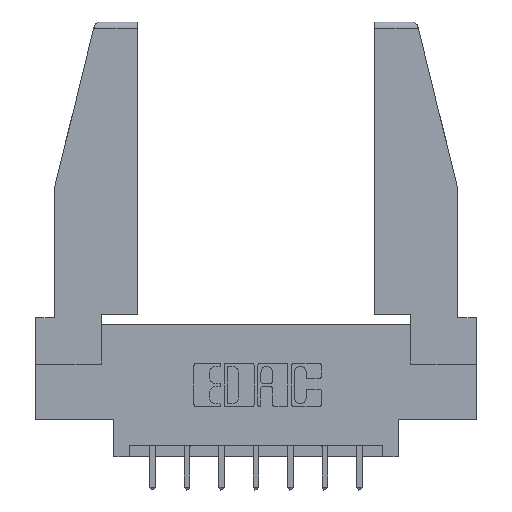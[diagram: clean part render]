
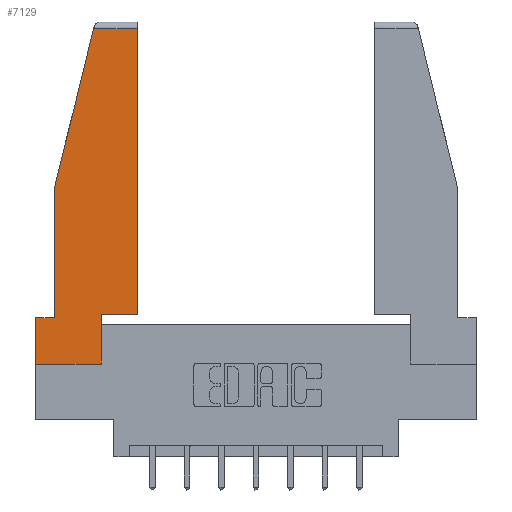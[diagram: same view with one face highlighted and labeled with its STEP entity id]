
A CAD part, top view. The second image highlights one B-rep face of the part: STEP entity #7129.
In plain terms, the highlighted planar face has unit normal (0, 0, 1).
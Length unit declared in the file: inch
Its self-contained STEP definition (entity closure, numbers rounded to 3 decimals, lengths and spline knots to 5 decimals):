
#118 = EDGE_CURVE ( 'NONE', #1076, #5311, #9170, .T. ) ;
#163 = VERTEX_POINT ( 'NONE', #5071 ) ;
#207 = VERTEX_POINT ( 'NONE', #1488 ) ;
#299 = VERTEX_POINT ( 'NONE', #12208 ) ;
#421 = CARTESIAN_POINT ( 'NONE',  ( 0.297, 0., 0. ) ) ;
#487 = VECTOR ( 'NONE', #8789, 39.37008 ) ;
#527 = AXIS2_PLACEMENT_3D ( 'NONE', #10409, #12367, #9402 ) ;
#644 = ORIENTED_EDGE ( 'NONE', *, *, #118, .T. ) ;
#921 = VERTEX_POINT ( 'NONE', #3981 ) ;
#1009 = ORIENTED_EDGE ( 'NONE', *, *, #2894, .T. ) ;
#1076 = VERTEX_POINT ( 'NONE', #8357 ) ;
#1488 = CARTESIAN_POINT ( 'NONE',  ( 0.297, 0., 0. ) ) ;
#1606 = VECTOR ( 'NONE', #11080, 39.37008 ) ;
#1769 = LINE ( 'NONE', #5513, #10834 ) ;
#1912 = VERTEX_POINT ( 'NONE', #5846 ) ;
#2113 = DIRECTION ( 'NONE',  ( 1., 0., 0. ) ) ;
#2365 = DIRECTION ( 'NONE',  ( 0., 1., 0. ) ) ;
#2510 = CARTESIAN_POINT ( 'NONE',  ( 0.461, 1.52, 0. ) ) ;
#2894 = EDGE_CURVE ( 'NONE', #207, #1076, #9684, .T. ) ;
#2986 = ORIENTED_EDGE ( 'NONE', *, *, #12083, .T. ) ;
#3292 = ORIENTED_EDGE ( 'NONE', *, *, #3628, .T. ) ;
#3396 = EDGE_CURVE ( 'NONE', #299, #207, #4759, .T. ) ;
#3402 = VECTOR ( 'NONE', #2113, 39.37008 ) ;
#3628 = EDGE_CURVE ( 'NONE', #163, #3728, #4744, .T. ) ;
#3660 = ORIENTED_EDGE ( 'NONE', *, *, #6737, .T. ) ;
#3682 = EDGE_CURVE ( 'NONE', #4040, #163, #1769, .T. ) ;
#3728 = VERTEX_POINT ( 'NONE', #12457 ) ;
#3729 = DIRECTION ( 'NONE',  ( -0.239, -0.971, 0. ) ) ;
#3820 = CARTESIAN_POINT ( 'NONE',  ( 0.461, 0.223, 0. ) ) ;
#3981 = CARTESIAN_POINT ( 'NONE',  ( 0.086, 0.21, 0. ) ) ;
#4040 = VERTEX_POINT ( 'NONE', #2510 ) ;
#4493 = VECTOR ( 'NONE', #2365, 39.37008 ) ;
#4611 = DIRECTION ( 'NONE',  ( -1., 0., 0. ) ) ;
#4672 = EDGE_CURVE ( 'NONE', #921, #1912, #11367, .T. ) ;
#4714 = ORIENTED_EDGE ( 'NONE', *, *, #8547, .T. ) ;
#4730 = FACE_OUTER_BOUND ( 'NONE', #9293, .T. ) ;
#4744 = LINE ( 'NONE', #6502, #12074 ) ;
#4759 = LINE ( 'NONE', #8992, #1606 ) ;
#5039 = LINE ( 'NONE', #6110, #5813 ) ;
#5071 = CARTESIAN_POINT ( 'NONE',  ( 0.2636, 1.52, 0. ) ) ;
#5252 = VECTOR ( 'NONE', #7064, 39.37008 ) ;
#5311 = VERTEX_POINT ( 'NONE', #9394 ) ;
#5513 = CARTESIAN_POINT ( 'NONE',  ( 0., 1.52, 0. ) ) ;
#5813 = VECTOR ( 'NONE', #12049, 39.37008 ) ;
#5846 = CARTESIAN_POINT ( 'NONE',  ( 0., 0.21, 0. ) ) ;
#6058 = LINE ( 'NONE', #3820, #487 ) ;
#6110 = CARTESIAN_POINT ( 'NONE',  ( 0.086, 0.8, 0. ) ) ;
#6320 = ORIENTED_EDGE ( 'NONE', *, *, #4672, .T. ) ;
#6502 = CARTESIAN_POINT ( 'NONE',  ( 0.271, 1.55, 0. ) ) ;
#6737 = EDGE_CURVE ( 'NONE', #3728, #921, #5039, .T. ) ;
#7064 = DIRECTION ( 'NONE',  ( 0., -1., 0. ) ) ;
#7129 = ADVANCED_FACE ( 'NONE', ( #4730 ), #12191, .T. ) ;
#7672 = DIRECTION ( 'NONE',  ( -1., 0., 0. ) ) ;
#8357 = CARTESIAN_POINT ( 'NONE',  ( 0.297, 0.223, 0. ) ) ;
#8547 = EDGE_CURVE ( 'NONE', #1912, #299, #12121, .T. ) ;
#8648 = VECTOR ( 'NONE', #4611, 39.37008 ) ;
#8789 = DIRECTION ( 'NONE',  ( 0., 1., 0. ) ) ;
#8992 = CARTESIAN_POINT ( 'NONE',  ( 0., 0., 0. ) ) ;
#9170 = LINE ( 'NONE', #11537, #3402 ) ;
#9293 = EDGE_LOOP ( 'NONE', ( #2986, #12253, #3292, #3660, #6320, #4714, #11620, #1009, #644 ) ) ;
#9394 = CARTESIAN_POINT ( 'NONE',  ( 0.461, 0.223, 0. ) ) ;
#9402 = DIRECTION ( 'NONE',  ( 1., 0., 0. ) ) ;
#9684 = LINE ( 'NONE', #421, #4493 ) ;
#10002 = CARTESIAN_POINT ( 'NONE',  ( 0., 0.21, 0. ) ) ;
#10409 = CARTESIAN_POINT ( 'NONE',  ( 0., 0., 0. ) ) ;
#10452 = CARTESIAN_POINT ( 'NONE',  ( 0., 0.21, 0. ) ) ;
#10834 = VECTOR ( 'NONE', #7672, 39.37008 ) ;
#11080 = DIRECTION ( 'NONE',  ( 1., 0., 0. ) ) ;
#11367 = LINE ( 'NONE', #10452, #8648 ) ;
#11537 = CARTESIAN_POINT ( 'NONE',  ( 0.297, 0.223, 0. ) ) ;
#11620 = ORIENTED_EDGE ( 'NONE', *, *, #3396, .T. ) ;
#12049 = DIRECTION ( 'NONE',  ( 0., -1., 0. ) ) ;
#12074 = VECTOR ( 'NONE', #3729, 39.37008 ) ;
#12083 = EDGE_CURVE ( 'NONE', #5311, #4040, #6058, .T. ) ;
#12121 = LINE ( 'NONE', #10002, #5252 ) ;
#12191 = PLANE ( 'NONE',  #527 ) ;
#12208 = CARTESIAN_POINT ( 'NONE',  ( 0., 0., 0. ) ) ;
#12253 = ORIENTED_EDGE ( 'NONE', *, *, #3682, .T. ) ;
#12367 = DIRECTION ( 'NONE',  ( 0., 0., 1. ) ) ;
#12457 = CARTESIAN_POINT ( 'NONE',  ( 0.086, 0.8, 0. ) ) ;
